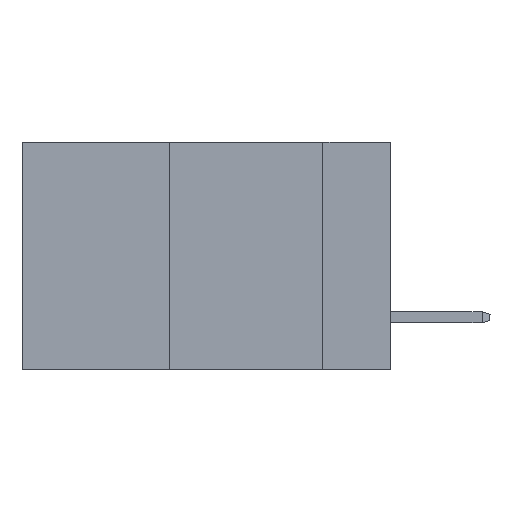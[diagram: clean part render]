
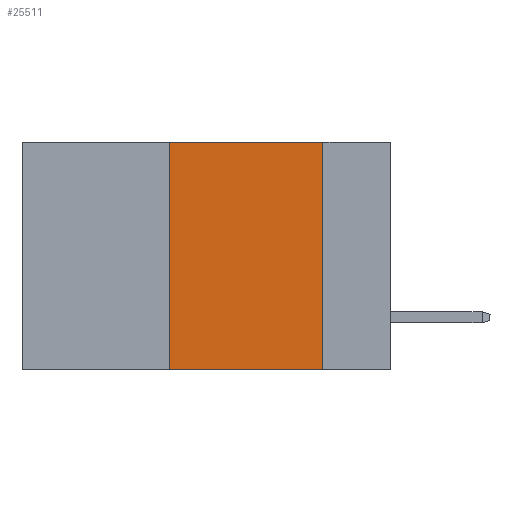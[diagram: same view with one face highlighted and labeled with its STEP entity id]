
A CAD part, left-side view. The second image highlights one B-rep face of the part: STEP entity #25511.
In plain terms, the highlighted planar face has unit normal (-1, 0, 0).
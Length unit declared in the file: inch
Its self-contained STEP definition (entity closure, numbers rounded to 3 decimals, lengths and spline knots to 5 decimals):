
#376 = LINE ( 'NONE', #14567, #18321 ) ;
#539 = DIRECTION ( 'NONE',  ( 0., -1., 0. ) ) ;
#703 = CARTESIAN_POINT ( 'NONE',  ( 0., 0.6, -0.37 ) ) ;
#1072 = DIRECTION ( 'NONE',  ( 0., -1., 0. ) ) ;
#1080 = EDGE_CURVE ( 'NONE', #17265, #1086, #12940, .T. ) ;
#1086 = VERTEX_POINT ( 'NONE', #5589 ) ;
#3526 = PLANE ( 'NONE',  #25035 ) ;
#4341 = VERTEX_POINT ( 'NONE', #14004 ) ;
#5105 = ORIENTED_EDGE ( 'NONE', *, *, #1080, .F. ) ;
#5108 = EDGE_CURVE ( 'NONE', #21016, #17265, #376, .T. ) ;
#5589 = CARTESIAN_POINT ( 'NONE',  ( 0., 0.11, -0.37 ) ) ;
#5846 = FACE_OUTER_BOUND ( 'NONE', #19221, .T. ) ;
#6515 = CARTESIAN_POINT ( 'NONE',  ( 0., 0.36, 0. ) ) ;
#7151 = DIRECTION ( 'NONE',  ( 1., 0., 0. ) ) ;
#7395 = CARTESIAN_POINT ( 'NONE',  ( 0., 0.11, 0. ) ) ;
#7795 = ORIENTED_EDGE ( 'NONE', *, *, #10543, .F. ) ;
#8081 = LINE ( 'NONE', #703, #11158 ) ;
#9398 = LINE ( 'NONE', #25276, #11875 ) ;
#10543 = EDGE_CURVE ( 'NONE', #4341, #21016, #9398, .T. ) ;
#11158 = VECTOR ( 'NONE', #539, 39.37008 ) ;
#11875 = VECTOR ( 'NONE', #17507, 39.37008 ) ;
#12940 = LINE ( 'NONE', #7395, #15447 ) ;
#13540 = DIRECTION ( 'NONE',  ( 0., 0., -1. ) ) ;
#14004 = CARTESIAN_POINT ( 'NONE',  ( 0., 0.36, -0.37 ) ) ;
#14567 = CARTESIAN_POINT ( 'NONE',  ( 0., 0.6, 0. ) ) ;
#14770 = EDGE_CURVE ( 'NONE', #4341, #1086, #8081, .T. ) ;
#15447 = VECTOR ( 'NONE', #13540, 39.37008 ) ;
#17126 = CARTESIAN_POINT ( 'NONE',  ( 0., 0.6, 0. ) ) ;
#17265 = VERTEX_POINT ( 'NONE', #21737 ) ;
#17380 = DIRECTION ( 'NONE',  ( 0., 0., -1. ) ) ;
#17507 = DIRECTION ( 'NONE',  ( 0., 0., 1. ) ) ;
#18321 = VECTOR ( 'NONE', #1072, 39.37008 ) ;
#19221 = EDGE_LOOP ( 'NONE', ( #5105, #20879, #7795, #22375 ) ) ;
#20879 = ORIENTED_EDGE ( 'NONE', *, *, #5108, .F. ) ;
#21016 = VERTEX_POINT ( 'NONE', #6515 ) ;
#21737 = CARTESIAN_POINT ( 'NONE',  ( 0., 0.11, 0. ) ) ;
#22375 = ORIENTED_EDGE ( 'NONE', *, *, #14770, .T. ) ;
#25035 = AXIS2_PLACEMENT_3D ( 'NONE', #17126, #7151, #17380 ) ;
#25276 = CARTESIAN_POINT ( 'NONE',  ( 0., 0.36, 0. ) ) ;
#25511 = ADVANCED_FACE ( 'NONE', ( #5846 ), #3526, .F. ) ;
